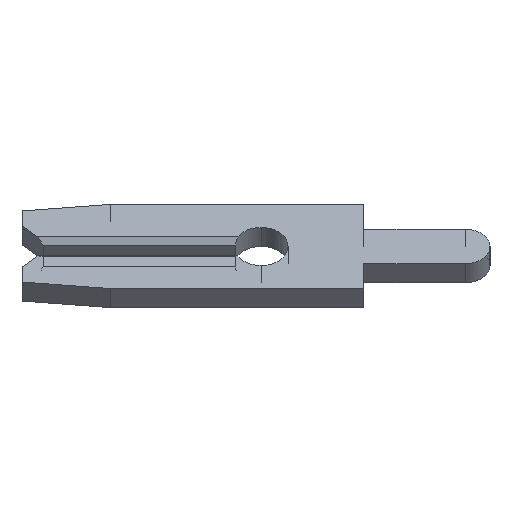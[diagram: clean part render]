
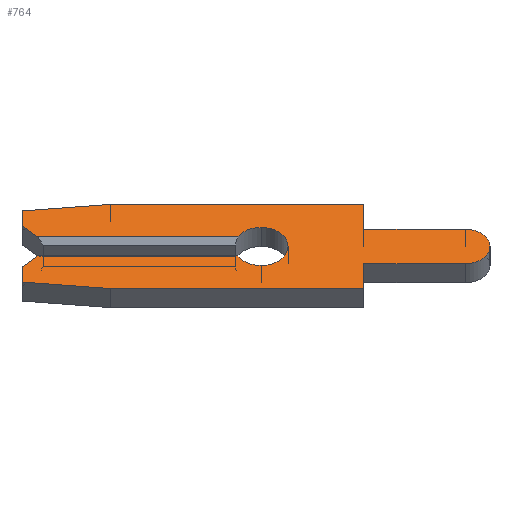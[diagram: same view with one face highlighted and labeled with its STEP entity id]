
A CAD part, left-side view. The second image highlights one B-rep face of the part: STEP entity #764.
In plain terms, the highlighted face is planar.
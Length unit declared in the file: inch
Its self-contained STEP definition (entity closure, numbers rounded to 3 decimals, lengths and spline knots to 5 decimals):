
#9 = VERTEX_POINT ( 'NONE', #314 ) ;
#24 = VECTOR ( 'NONE', #997, 39.37008 ) ;
#30 = EDGE_CURVE ( 'NONE', #675, #920, #1113, .T. ) ;
#37 = DIRECTION ( 'NONE',  ( 0., -1., 0. ) ) ;
#42 = CARTESIAN_POINT ( 'NONE',  ( -0.013, 0., 0.026 ) ) ;
#62 = AXIS2_PLACEMENT_3D ( 'NONE', #1061, #172, #1929 ) ;
#66 = CARTESIAN_POINT ( 'NONE',  ( -0.013, 0., -0.013 ) ) ;
#76 = ORIENTED_EDGE ( 'NONE', *, *, #178, .F. ) ;
#85 = CARTESIAN_POINT ( 'NONE',  ( -0.013, 0.216, -0.013 ) ) ;
#102 = LINE ( 'NONE', #1093, #1100 ) ;
#112 = VECTOR ( 'NONE', #1824, 39.37008 ) ;
#140 = LINE ( 'NONE', #1404, #2042 ) ;
#158 = LINE ( 'NONE', #459, #446 ) ;
#163 = VECTOR ( 'NONE', #1112, 39.37008 ) ;
#172 = DIRECTION ( 'NONE',  ( -1., 0., 0. ) ) ;
#178 = EDGE_CURVE ( 'NONE', #266, #1534, #1308, .T. ) ;
#198 = EDGE_CURVE ( 'NONE', #714, #608, #2011, .T. ) ;
#215 = CARTESIAN_POINT ( 'NONE',  ( -0.013, 0.231, 0.013 ) ) ;
#218 = CIRCLE ( 'NONE', #850, 0.026 ) ;
#229 = EDGE_CURVE ( 'NONE', #743, #9, #2155, .T. ) ;
#266 = VERTEX_POINT ( 'NONE', #1236 ) ;
#305 = LINE ( 'NONE', #215, #1201 ) ;
#314 = CARTESIAN_POINT ( 'NONE',  ( -0.013, -0.099, -0.0575 ) ) ;
#334 = DIRECTION ( 'NONE',  ( 0., 0., -1. ) ) ;
#342 = DIRECTION ( 'NONE',  ( 0., 0., 1. ) ) ;
#348 = ORIENTED_EDGE ( 'NONE', *, *, #1597, .F. ) ;
#354 = ORIENTED_EDGE ( 'NONE', *, *, #431, .F. ) ;
#387 = ORIENTED_EDGE ( 'NONE', *, *, #1522, .F. ) ;
#397 = EDGE_CURVE ( 'NONE', #2050, #743, #140, .T. ) ;
#400 = CARTESIAN_POINT ( 'NONE',  ( -0.013, 0., 0. ) ) ;
#402 = VERTEX_POINT ( 'NONE', #1925 ) ;
#408 = CARTESIAN_POINT ( 'NONE',  ( -0.013, -0.099, 0.0575 ) ) ;
#409 = ORIENTED_EDGE ( 'NONE', *, *, #870, .F. ) ;
#426 = DIRECTION ( 'NONE',  ( 0., 0.707, 0.707 ) ) ;
#431 = EDGE_CURVE ( 'NONE', #1091, #1806, #1335, .T. ) ;
#434 = CARTESIAN_POINT ( 'NONE',  ( -0.013, 0.231, 0.04857 ) ) ;
#446 = VECTOR ( 'NONE', #2099, 39.37008 ) ;
#447 = ORIENTED_EDGE ( 'NONE', *, *, #681, .F. ) ;
#453 = CARTESIAN_POINT ( 'NONE',  ( -0.013, -0.1975, 0.0235 ) ) ;
#456 = VERTEX_POINT ( 'NONE', #1047 ) ;
#459 = CARTESIAN_POINT ( 'NONE',  ( -0.013, 0.231, -0.04857 ) ) ;
#474 = ORIENTED_EDGE ( 'NONE', *, *, #1107, .F. ) ;
#476 = LINE ( 'NONE', #931, #112 ) ;
#484 = CARTESIAN_POINT ( 'NONE',  ( -0.013, 0.231, 0.028 ) ) ;
#522 = DIRECTION ( 'NONE',  ( -1., 0., 0. ) ) ;
#538 = DIRECTION ( 'NONE',  ( 0., 0., -1. ) ) ;
#540 = CARTESIAN_POINT ( 'NONE',  ( -0.013, -0.1975, 0. ) ) ;
#561 = ORIENTED_EDGE ( 'NONE', *, *, #1019, .F. ) ;
#566 = DIRECTION ( 'NONE',  ( 0., 0., 1. ) ) ;
#571 = AXIS2_PLACEMENT_3D ( 'NONE', #1763, #522, #538 ) ;
#595 = CARTESIAN_POINT ( 'NONE',  ( -0.013, -0.099, 0.0575 ) ) ;
#608 = VERTEX_POINT ( 'NONE', #900 ) ;
#627 = CARTESIAN_POINT ( 'NONE',  ( -0.013, 0.231, 0.04857 ) ) ;
#642 = VECTOR ( 'NONE', #37, 39.37008 ) ;
#648 = CARTESIAN_POINT ( 'NONE',  ( -0.013, 0.146, 0.0575 ) ) ;
#664 = CIRCLE ( 'NONE', #1886, 0.0235 ) ;
#666 = EDGE_CURVE ( 'NONE', #1534, #714, #218, .T. ) ;
#675 = VERTEX_POINT ( 'NONE', #1443 ) ;
#681 = EDGE_CURVE ( 'NONE', #1405, #1395, #1171, .T. ) ;
#714 = VERTEX_POINT ( 'NONE', #42 ) ;
#719 = LINE ( 'NONE', #1494, #1513 ) ;
#736 = PLANE ( 'NONE',  #1668 ) ;
#743 = VERTEX_POINT ( 'NONE', #1985 ) ;
#764 = ADVANCED_FACE ( 'NONE', ( #831 ), #736, .F. ) ;
#783 = EDGE_CURVE ( 'NONE', #456, #608, #305, .T. ) ;
#831 = FACE_OUTER_BOUND ( 'NONE', #2192, .T. ) ;
#849 = LINE ( 'NONE', #627, #910 ) ;
#850 = AXIS2_PLACEMENT_3D ( 'NONE', #1260, #927, #894 ) ;
#858 = VECTOR ( 'NONE', #1935, 39.37008 ) ;
#870 = EDGE_CURVE ( 'NONE', #456, #675, #719, .T. ) ;
#874 = CARTESIAN_POINT ( 'NONE',  ( -0.013, 0.231, -0.028 ) ) ;
#894 = DIRECTION ( 'NONE',  ( 0., 0., -1. ) ) ;
#900 = CARTESIAN_POINT ( 'NONE',  ( -0.013, 0.02252, 0.013 ) ) ;
#910 = VECTOR ( 'NONE', #1154, 39.37008 ) ;
#912 = CARTESIAN_POINT ( 'NONE',  ( -0.013, -0.1975, -0.0235 ) ) ;
#918 = VECTOR ( 'NONE', #342, 39.37008 ) ;
#920 = VERTEX_POINT ( 'NONE', #434 ) ;
#927 = DIRECTION ( 'NONE',  ( -1., 0., 0. ) ) ;
#931 = CARTESIAN_POINT ( 'NONE',  ( -0.013, 0.2105, -0.0075 ) ) ;
#948 = LINE ( 'NONE', #66, #642 ) ;
#986 = EDGE_CURVE ( 'NONE', #1806, #1607, #476, .T. ) ;
#997 = DIRECTION ( 'NONE',  ( 0., 0., 1. ) ) ;
#999 = LINE ( 'NONE', #595, #163 ) ;
#1019 = EDGE_CURVE ( 'NONE', #2145, #1405, #999, .T. ) ;
#1037 = ORIENTED_EDGE ( 'NONE', *, *, #397, .F. ) ;
#1044 = ORIENTED_EDGE ( 'NONE', *, *, #229, .F. ) ;
#1047 = CARTESIAN_POINT ( 'NONE',  ( -0.013, 0.216, 0.013 ) ) ;
#1060 = EDGE_CURVE ( 'NONE', #1607, #266, #948, .T. ) ;
#1061 = CARTESIAN_POINT ( 'NONE',  ( -0.013, 0., 0. ) ) ;
#1082 = ORIENTED_EDGE ( 'NONE', *, *, #986, .F. ) ;
#1091 = VERTEX_POINT ( 'NONE', #2211 ) ;
#1093 = CARTESIAN_POINT ( 'NONE',  ( -0.013, 0.146, -0.0575 ) ) ;
#1095 = ORIENTED_EDGE ( 'NONE', *, *, #1060, .F. ) ;
#1100 = VECTOR ( 'NONE', #1993, 39.37008 ) ;
#1107 = EDGE_CURVE ( 'NONE', #1508, #2145, #1481, .T. ) ;
#1112 = DIRECTION ( 'NONE',  ( 0., 0., -1. ) ) ;
#1113 = LINE ( 'NONE', #484, #24 ) ;
#1147 = CARTESIAN_POINT ( 'NONE',  ( -0.013, 0.146, 0.0575 ) ) ;
#1154 = DIRECTION ( 'NONE',  ( 0., -0.995, 0.105 ) ) ;
#1171 = LINE ( 'NONE', #2152, #2236 ) ;
#1201 = VECTOR ( 'NONE', #1653, 39.37008 ) ;
#1236 = CARTESIAN_POINT ( 'NONE',  ( -0.013, 0.02252, -0.013 ) ) ;
#1260 = CARTESIAN_POINT ( 'NONE',  ( -0.013, 0., 0. ) ) ;
#1308 = CIRCLE ( 'NONE', #571, 0.026 ) ;
#1335 = LINE ( 'NONE', #874, #918 ) ;
#1395 = VERTEX_POINT ( 'NONE', #453 ) ;
#1397 = DIRECTION ( 'NONE',  ( 0., 1., 0. ) ) ;
#1404 = CARTESIAN_POINT ( 'NONE',  ( -0.013, -0.099, -0.0235 ) ) ;
#1405 = VERTEX_POINT ( 'NONE', #2261 ) ;
#1413 = ORIENTED_EDGE ( 'NONE', *, *, #666, .F. ) ;
#1432 = DIRECTION ( 'NONE',  ( 1., 0., 0. ) ) ;
#1443 = CARTESIAN_POINT ( 'NONE',  ( -0.013, 0.231, 0.028 ) ) ;
#1481 = LINE ( 'NONE', #1147, #1894 ) ;
#1494 = CARTESIAN_POINT ( 'NONE',  ( -0.013, 0.2105, 0.0075 ) ) ;
#1508 = VERTEX_POINT ( 'NONE', #648 ) ;
#1513 = VECTOR ( 'NONE', #426, 39.37008 ) ;
#1522 = EDGE_CURVE ( 'NONE', #920, #1508, #849, .T. ) ;
#1534 = VERTEX_POINT ( 'NONE', #1709 ) ;
#1544 = ORIENTED_EDGE ( 'NONE', *, *, #1871, .F. ) ;
#1585 = CARTESIAN_POINT ( 'NONE',  ( -0.013, -0.099, -0.0575 ) ) ;
#1597 = EDGE_CURVE ( 'NONE', #402, #1091, #158, .T. ) ;
#1607 = VERTEX_POINT ( 'NONE', #85 ) ;
#1611 = ORIENTED_EDGE ( 'NONE', *, *, #198, .F. ) ;
#1653 = DIRECTION ( 'NONE',  ( 0., -1., 0. ) ) ;
#1654 = ORIENTED_EDGE ( 'NONE', *, *, #30, .F. ) ;
#1668 = AXIS2_PLACEMENT_3D ( 'NONE', #400, #1432, #334 ) ;
#1709 = CARTESIAN_POINT ( 'NONE',  ( -0.013, 0., -0.026 ) ) ;
#1763 = CARTESIAN_POINT ( 'NONE',  ( -0.013, 0., 0. ) ) ;
#1791 = DIRECTION ( 'NONE',  ( 0., -1., 0. ) ) ;
#1806 = VERTEX_POINT ( 'NONE', #1909 ) ;
#1824 = DIRECTION ( 'NONE',  ( 0., -0.707, 0.707 ) ) ;
#1871 = EDGE_CURVE ( 'NONE', #9, #402, #102, .T. ) ;
#1886 = AXIS2_PLACEMENT_3D ( 'NONE', #540, #1960, #566 ) ;
#1894 = VECTOR ( 'NONE', #2191, 39.37008 ) ;
#1909 = CARTESIAN_POINT ( 'NONE',  ( -0.013, 0.231, -0.028 ) ) ;
#1925 = CARTESIAN_POINT ( 'NONE',  ( -0.013, 0.146, -0.0575 ) ) ;
#1929 = DIRECTION ( 'NONE',  ( 0., 0., -1. ) ) ;
#1935 = DIRECTION ( 'NONE',  ( 0., 0., -1. ) ) ;
#1949 = ORIENTED_EDGE ( 'NONE', *, *, #2025, .F. ) ;
#1960 = DIRECTION ( 'NONE',  ( 1., 0., 0. ) ) ;
#1985 = CARTESIAN_POINT ( 'NONE',  ( -0.013, -0.099, -0.0235 ) ) ;
#1993 = DIRECTION ( 'NONE',  ( 0., 1., 0. ) ) ;
#2011 = CIRCLE ( 'NONE', #62, 0.026 ) ;
#2025 = EDGE_CURVE ( 'NONE', #1395, #2050, #664, .T. ) ;
#2042 = VECTOR ( 'NONE', #1397, 39.37008 ) ;
#2050 = VERTEX_POINT ( 'NONE', #912 ) ;
#2073 = ORIENTED_EDGE ( 'NONE', *, *, #783, .T. ) ;
#2099 = DIRECTION ( 'NONE',  ( 0., 0.995, 0.105 ) ) ;
#2145 = VERTEX_POINT ( 'NONE', #408 ) ;
#2152 = CARTESIAN_POINT ( 'NONE',  ( -0.013, -0.099, 0.0235 ) ) ;
#2155 = LINE ( 'NONE', #1585, #858 ) ;
#2191 = DIRECTION ( 'NONE',  ( 0., -1., 0. ) ) ;
#2192 = EDGE_LOOP ( 'NONE', ( #2073, #1611, #1413, #76, #1095, #1082, #354, #348, #1544, #1044, #1037, #1949, #447, #561, #474, #387, #1654, #409 ) ) ;
#2211 = CARTESIAN_POINT ( 'NONE',  ( -0.013, 0.231, -0.04857 ) ) ;
#2236 = VECTOR ( 'NONE', #1791, 39.37008 ) ;
#2261 = CARTESIAN_POINT ( 'NONE',  ( -0.013, -0.099, 0.0235 ) ) ;
